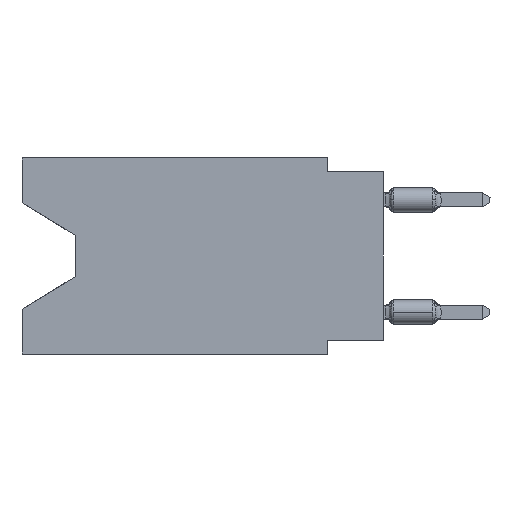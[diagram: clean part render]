
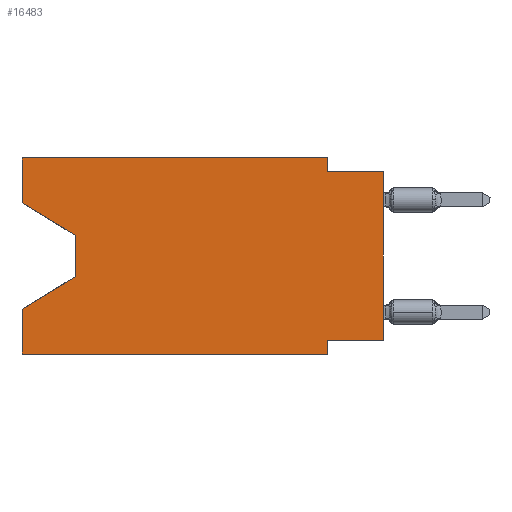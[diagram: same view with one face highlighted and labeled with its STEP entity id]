
A CAD part, left-side view. The second image highlights one B-rep face of the part: STEP entity #16483.
In plain terms, the highlighted planar face has unit normal (-1, 0, 0).
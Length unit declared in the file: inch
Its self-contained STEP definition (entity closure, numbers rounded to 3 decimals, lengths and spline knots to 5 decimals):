
#93 = DIRECTION ( 'NONE',  ( 0., 0., 1. ) ) ;
#109 = VECTOR ( 'NONE', #25802, 39.37008 ) ;
#304 = EDGE_CURVE ( 'NONE', #975, #589, #21027, .T. ) ;
#377 = EDGE_CURVE ( 'NONE', #25320, #25025, #10176, .T. ) ;
#589 = VERTEX_POINT ( 'NONE', #12828 ) ;
#695 = CARTESIAN_POINT ( 'NONE',  ( 0., 0.1, -0.35 ) ) ;
#844 = EDGE_CURVE ( 'NONE', #8451, #27862, #28138, .T. ) ;
#925 = DIRECTION ( 'NONE',  ( 0., -1., 0. ) ) ;
#975 = VERTEX_POINT ( 'NONE', #28427 ) ;
#1040 = CARTESIAN_POINT ( 'NONE',  ( 0., 0.1, -0.325 ) ) ;
#1162 = CARTESIAN_POINT ( 'NONE',  ( 0., 0.55, -0.212 ) ) ;
#1248 = CARTESIAN_POINT ( 'NONE',  ( 0., 0.1, -0.025 ) ) ;
#1699 = VERTEX_POINT ( 'NONE', #4130 ) ;
#2426 = DIRECTION ( 'NONE',  ( 0., 0.855, -0.519 ) ) ;
#2431 = CARTESIAN_POINT ( 'NONE',  ( 0., 0.55, -0.138 ) ) ;
#2495 = LINE ( 'NONE', #4445, #3502 ) ;
#2568 = LINE ( 'NONE', #6765, #22238 ) ;
#3502 = VECTOR ( 'NONE', #9496, 39.37008 ) ;
#3527 = VERTEX_POINT ( 'NONE', #1162 ) ;
#3593 = CARTESIAN_POINT ( 'NONE',  ( 0., 0.1, 0. ) ) ;
#3960 = DIRECTION ( 'NONE',  ( 0., 0., 1. ) ) ;
#4130 = CARTESIAN_POINT ( 'NONE',  ( 0., 0.645, -0.26975 ) ) ;
#4425 = ORIENTED_EDGE ( 'NONE', *, *, #377, .F. ) ;
#4445 = CARTESIAN_POINT ( 'NONE',  ( 0., 0.645, 0. ) ) ;
#4542 = VECTOR ( 'NONE', #23295, 39.37008 ) ;
#4797 = DIRECTION ( 'NONE',  ( 0., 0., -1. ) ) ;
#5099 = CARTESIAN_POINT ( 'NONE',  ( 0., 0.645, 0. ) ) ;
#5396 = DIRECTION ( 'NONE',  ( 0., 0., 1. ) ) ;
#6204 = LINE ( 'NONE', #15269, #22534 ) ;
#6765 = CARTESIAN_POINT ( 'NONE',  ( 0., 0.645, -0.08025 ) ) ;
#7278 = DIRECTION ( 'NONE',  ( 0., 0., -1. ) ) ;
#7355 = VERTEX_POINT ( 'NONE', #8599 ) ;
#7494 = PLANE ( 'NONE',  #8850 ) ;
#7651 = CARTESIAN_POINT ( 'NONE',  ( 0., 0.645, -0.35 ) ) ;
#7665 = VECTOR ( 'NONE', #5396, 39.37008 ) ;
#8188 = CARTESIAN_POINT ( 'NONE',  ( 0., 0., -0.025 ) ) ;
#8424 = ORIENTED_EDGE ( 'NONE', *, *, #27414, .T. ) ;
#8451 = VERTEX_POINT ( 'NONE', #26480 ) ;
#8599 = CARTESIAN_POINT ( 'NONE',  ( 0., 0.645, 0. ) ) ;
#8850 = AXIS2_PLACEMENT_3D ( 'NONE', #25491, #27569, #4797 ) ;
#9124 = EDGE_CURVE ( 'NONE', #27862, #589, #23310, .T. ) ;
#9425 = DIRECTION ( 'NONE',  ( 0., -0.855, -0.519 ) ) ;
#9496 = DIRECTION ( 'NONE',  ( 0., -1., 0. ) ) ;
#9850 = VERTEX_POINT ( 'NONE', #3593 ) ;
#10176 = LINE ( 'NONE', #16424, #17702 ) ;
#11718 = EDGE_CURVE ( 'NONE', #975, #1699, #20918, .T. ) ;
#12156 = CARTESIAN_POINT ( 'NONE',  ( 0., 0.645, 0. ) ) ;
#12621 = ORIENTED_EDGE ( 'NONE', *, *, #26355, .F. ) ;
#12828 = CARTESIAN_POINT ( 'NONE',  ( 0., 0.1, -0.35 ) ) ;
#13462 = CARTESIAN_POINT ( 'NONE',  ( 0., 0.55, -0.212 ) ) ;
#13488 = VERTEX_POINT ( 'NONE', #2431 ) ;
#14392 = ORIENTED_EDGE ( 'NONE', *, *, #28876, .T. ) ;
#14921 = EDGE_CURVE ( 'NONE', #9850, #25320, #25098, .T. ) ;
#14999 = ORIENTED_EDGE ( 'NONE', *, *, #23491, .F. ) ;
#15269 = CARTESIAN_POINT ( 'NONE',  ( 0., 0., 0. ) ) ;
#15883 = VECTOR ( 'NONE', #2426, 39.37008 ) ;
#16184 = VECTOR ( 'NONE', #7278, 39.37008 ) ;
#16412 = FACE_OUTER_BOUND ( 'NONE', #21526, .T. ) ;
#16424 = CARTESIAN_POINT ( 'NONE',  ( 0., 0., -0.025 ) ) ;
#16445 = DIRECTION ( 'NONE',  ( 0., 0., -1. ) ) ;
#16483 = ADVANCED_FACE ( 'NONE', ( #16412 ), #7494, .F. ) ;
#17340 = VERTEX_POINT ( 'NONE', #23339 ) ;
#17702 = VECTOR ( 'NONE', #925, 39.37008 ) ;
#18059 = ORIENTED_EDGE ( 'NONE', *, *, #11718, .F. ) ;
#19890 = VECTOR ( 'NONE', #16445, 39.37008 ) ;
#20193 = EDGE_CURVE ( 'NONE', #13488, #3527, #27759, .T. ) ;
#20770 = ORIENTED_EDGE ( 'NONE', *, *, #304, .T. ) ;
#20896 = CARTESIAN_POINT ( 'NONE',  ( 0., 0.55, -0.138 ) ) ;
#20918 = LINE ( 'NONE', #12156, #28113 ) ;
#20985 = CARTESIAN_POINT ( 'NONE',  ( 0., 0., -0.325 ) ) ;
#21027 = LINE ( 'NONE', #7651, #109 ) ;
#21526 = EDGE_LOOP ( 'NONE', ( #14392, #26027, #8424, #18059, #20770, #23176, #28483, #22680, #4425, #25659, #12621, #14999 ) ) ;
#22238 = VECTOR ( 'NONE', #9425, 39.37008 ) ;
#22534 = VECTOR ( 'NONE', #3960, 39.37008 ) ;
#22680 = ORIENTED_EDGE ( 'NONE', *, *, #26626, .T. ) ;
#22714 = CARTESIAN_POINT ( 'NONE',  ( 0., 0.1, 0. ) ) ;
#22957 = LINE ( 'NONE', #13462, #15883 ) ;
#23176 = ORIENTED_EDGE ( 'NONE', *, *, #9124, .F. ) ;
#23295 = DIRECTION ( 'NONE',  ( 0., 0., -1. ) ) ;
#23310 = LINE ( 'NONE', #695, #16184 ) ;
#23339 = CARTESIAN_POINT ( 'NONE',  ( 0., 0.645, -0.08025 ) ) ;
#23491 = EDGE_CURVE ( 'NONE', #17340, #7355, #25503, .T. ) ;
#23887 = VECTOR ( 'NONE', #27705, 39.37008 ) ;
#25025 = VERTEX_POINT ( 'NONE', #8188 ) ;
#25098 = LINE ( 'NONE', #22714, #4542 ) ;
#25320 = VERTEX_POINT ( 'NONE', #1248 ) ;
#25491 = CARTESIAN_POINT ( 'NONE',  ( 0., 0.645, 0. ) ) ;
#25503 = LINE ( 'NONE', #5099, #7665 ) ;
#25659 = ORIENTED_EDGE ( 'NONE', *, *, #14921, .F. ) ;
#25802 = DIRECTION ( 'NONE',  ( 0., -1., 0. ) ) ;
#26027 = ORIENTED_EDGE ( 'NONE', *, *, #20193, .T. ) ;
#26355 = EDGE_CURVE ( 'NONE', #7355, #9850, #2495, .T. ) ;
#26480 = CARTESIAN_POINT ( 'NONE',  ( 0., 0., -0.325 ) ) ;
#26626 = EDGE_CURVE ( 'NONE', #8451, #25025, #6204, .T. ) ;
#27414 = EDGE_CURVE ( 'NONE', #3527, #1699, #22957, .T. ) ;
#27569 = DIRECTION ( 'NONE',  ( 1., 0., 0. ) ) ;
#27705 = DIRECTION ( 'NONE',  ( 0., 1., 0. ) ) ;
#27759 = LINE ( 'NONE', #20896, #19890 ) ;
#27862 = VERTEX_POINT ( 'NONE', #1040 ) ;
#28113 = VECTOR ( 'NONE', #93, 39.37008 ) ;
#28138 = LINE ( 'NONE', #20985, #23887 ) ;
#28427 = CARTESIAN_POINT ( 'NONE',  ( 0., 0.645, -0.35 ) ) ;
#28483 = ORIENTED_EDGE ( 'NONE', *, *, #844, .F. ) ;
#28876 = EDGE_CURVE ( 'NONE', #17340, #13488, #2568, .T. ) ;
